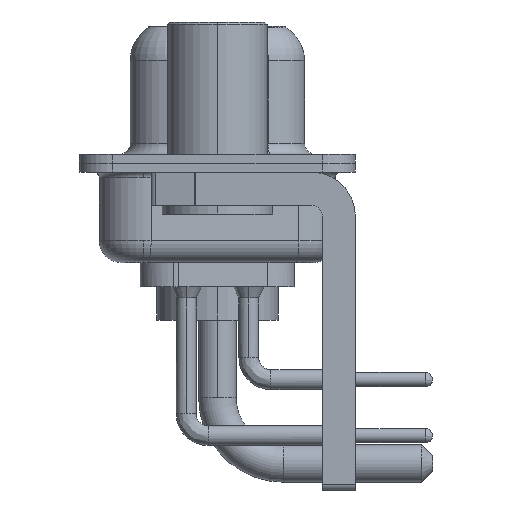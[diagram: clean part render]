
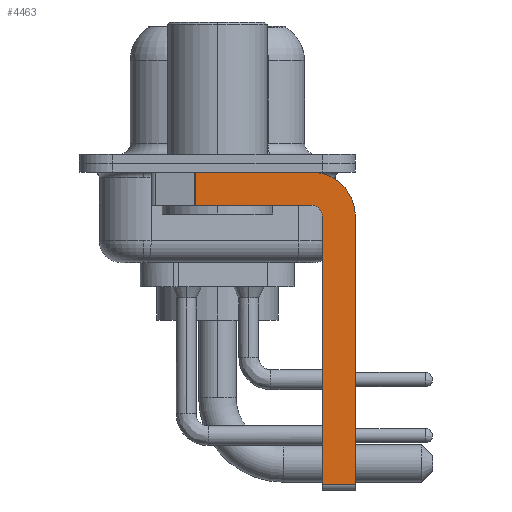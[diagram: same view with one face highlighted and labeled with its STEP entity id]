
A CAD part, left-side view. The second image highlights one B-rep face of the part: STEP entity #4463.
In plain terms, the highlighted planar face has unit normal (-1, 0, 0).
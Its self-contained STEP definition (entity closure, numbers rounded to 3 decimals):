
#57 = LINE ( 'NONE', #9947, #1514 ) ;
#265 = VECTOR ( 'NONE', #5322, 1000. ) ;
#379 = DIRECTION ( 'NONE',  ( 0., 0., -1. ) ) ;
#406 = DIRECTION ( 'NONE',  ( 0., 1., 0. ) ) ;
#656 = FACE_OUTER_BOUND ( 'NONE', #6699, .T. ) ;
#1129 = CARTESIAN_POINT ( 'NONE',  ( -2.9, -4.75, -2.4 ) ) ;
#1403 = CARTESIAN_POINT ( 'NONE',  ( -2.9, 3., -0.4 ) ) ;
#1514 = VECTOR ( 'NONE', #15856, 1000. ) ;
#1558 = VERTEX_POINT ( 'NONE', #14470 ) ;
#1577 = CARTESIAN_POINT ( 'NONE',  ( -2.9, -4.75, -14.55 ) ) ;
#1736 = CARTESIAN_POINT ( 'NONE',  ( -2.9, -4.25, -1.9 ) ) ;
#1739 = VERTEX_POINT ( 'NONE', #13889 ) ;
#2227 = ORIENTED_EDGE ( 'NONE', *, *, #13076, .F. ) ;
#2779 = EDGE_CURVE ( 'NONE', #11364, #11434, #57, .T. ) ;
#3347 = AXIS2_PLACEMENT_3D ( 'NONE', #11312, #4375, #14263 ) ;
#3523 = CARTESIAN_POINT ( 'NONE',  ( -2.9, -4.75, -14.8 ) ) ;
#3599 = PLANE ( 'NONE',  #9030 ) ;
#4169 = CARTESIAN_POINT ( 'NONE',  ( -2.9, 0.978, -1.9 ) ) ;
#4375 = DIRECTION ( 'NONE',  ( -1., 0., 0. ) ) ;
#4463 = ADVANCED_FACE ( 'NONE', ( #656 ), #3599, .F. ) ;
#5322 = DIRECTION ( 'NONE',  ( 0., 0., -1. ) ) ;
#5810 = AXIS2_PLACEMENT_3D ( 'NONE', #8851, #12928, #14560 ) ;
#5847 = EDGE_CURVE ( 'NONE', #9567, #1739, #16495, .T. ) ;
#6066 = ORIENTED_EDGE ( 'NONE', *, *, #2779, .T. ) ;
#6263 = DIRECTION ( 'NONE',  ( 0., 0., 1. ) ) ;
#6468 = ORIENTED_EDGE ( 'NONE', *, *, #16611, .F. ) ;
#6699 = EDGE_LOOP ( 'NONE', ( #6468, #7066, #16555, #14137, #15865, #6066, #2227, #18811 ) ) ;
#7066 = ORIENTED_EDGE ( 'NONE', *, *, #7737, .T. ) ;
#7484 = EDGE_CURVE ( 'NONE', #11364, #10809, #13701, .T. ) ;
#7587 = CARTESIAN_POINT ( 'NONE',  ( -2.9, -4.25, -2.4 ) ) ;
#7737 = EDGE_CURVE ( 'NONE', #1558, #16387, #11492, .T. ) ;
#8634 = DIRECTION ( 'NONE',  ( 0., 0., -1. ) ) ;
#8851 = CARTESIAN_POINT ( 'NONE',  ( -2.9, -4.25, -2.4 ) ) ;
#9030 = AXIS2_PLACEMENT_3D ( 'NONE', #7587, #15216, #379 ) ;
#9239 = CARTESIAN_POINT ( 'NONE',  ( -2.9, -4.25, -1.9 ) ) ;
#9567 = VERTEX_POINT ( 'NONE', #10433 ) ;
#9681 = CARTESIAN_POINT ( 'NONE',  ( -2.9, 0.978, -1.9 ) ) ;
#9947 = CARTESIAN_POINT ( 'NONE',  ( -2.9, -4.25, -14.55 ) ) ;
#10007 = CIRCLE ( 'NONE', #3347, 0.5 ) ;
#10433 = CARTESIAN_POINT ( 'NONE',  ( -2.9, -4.25, -0.4 ) ) ;
#10468 = LINE ( 'NONE', #9239, #11277 ) ;
#10809 = VERTEX_POINT ( 'NONE', #1129 ) ;
#11277 = VECTOR ( 'NONE', #406, 1000. ) ;
#11312 = CARTESIAN_POINT ( 'NONE',  ( -2.9, -4.25, -2.4 ) ) ;
#11364 = VERTEX_POINT ( 'NONE', #1577 ) ;
#11434 = VERTEX_POINT ( 'NONE', #17475 ) ;
#11492 = LINE ( 'NONE', #4169, #18687 ) ;
#12570 = CARTESIAN_POINT ( 'NONE',  ( -2.9, -6.25, -2.4 ) ) ;
#12904 = DIRECTION ( 'NONE',  ( 0., -1., 0. ) ) ;
#12928 = DIRECTION ( 'NONE',  ( 1., 0., 0. ) ) ;
#13076 = EDGE_CURVE ( 'NONE', #1739, #11434, #17059, .T. ) ;
#13701 = LINE ( 'NONE', #3523, #14730 ) ;
#13889 = CARTESIAN_POINT ( 'NONE',  ( -2.9, -6.25, -2.4 ) ) ;
#14137 = ORIENTED_EDGE ( 'NONE', *, *, #16096, .F. ) ;
#14263 = DIRECTION ( 'NONE',  ( 0., 0., 1. ) ) ;
#14470 = CARTESIAN_POINT ( 'NONE',  ( -2.9, 0.978, -0.4 ) ) ;
#14560 = DIRECTION ( 'NONE',  ( 0., 0., -1. ) ) ;
#14730 = VECTOR ( 'NONE', #6263, 1000. ) ;
#15216 = DIRECTION ( 'NONE',  ( 1., 0., 0. ) ) ;
#15849 = VERTEX_POINT ( 'NONE', #1736 ) ;
#15856 = DIRECTION ( 'NONE',  ( 0., -1., 0. ) ) ;
#15865 = ORIENTED_EDGE ( 'NONE', *, *, #7484, .F. ) ;
#16096 = EDGE_CURVE ( 'NONE', #10809, #15849, #10007, .T. ) ;
#16387 = VERTEX_POINT ( 'NONE', #9681 ) ;
#16495 = CIRCLE ( 'NONE', #5810, 2. ) ;
#16555 = ORIENTED_EDGE ( 'NONE', *, *, #17946, .F. ) ;
#16611 = EDGE_CURVE ( 'NONE', #1558, #9567, #18450, .T. ) ;
#17059 = LINE ( 'NONE', #12570, #265 ) ;
#17336 = VECTOR ( 'NONE', #12904, 1000. ) ;
#17475 = CARTESIAN_POINT ( 'NONE',  ( -2.9, -6.25, -14.55 ) ) ;
#17946 = EDGE_CURVE ( 'NONE', #15849, #16387, #10468, .T. ) ;
#18450 = LINE ( 'NONE', #1403, #17336 ) ;
#18687 = VECTOR ( 'NONE', #8634, 1000. ) ;
#18811 = ORIENTED_EDGE ( 'NONE', *, *, #5847, .F. ) ;
